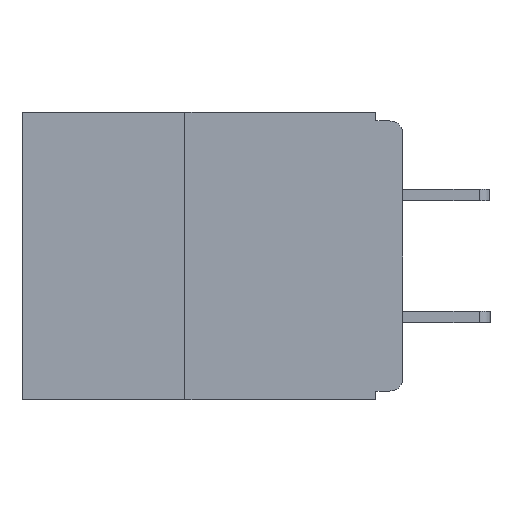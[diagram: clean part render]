
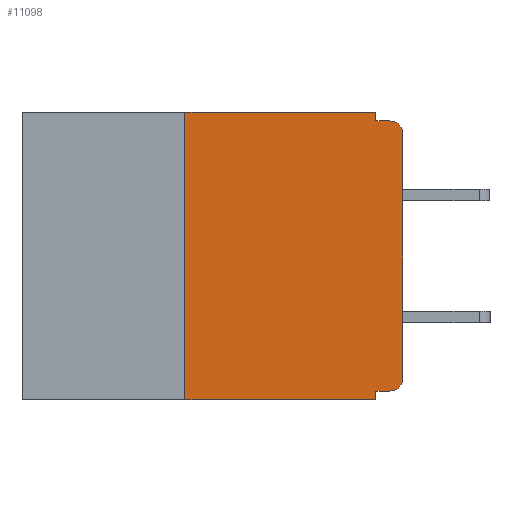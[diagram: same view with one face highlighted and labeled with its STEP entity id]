
A CAD part, left-side view. The second image highlights one B-rep face of the part: STEP entity #11098.
In plain terms, the highlighted planar face has unit normal (-1, 0, 0).
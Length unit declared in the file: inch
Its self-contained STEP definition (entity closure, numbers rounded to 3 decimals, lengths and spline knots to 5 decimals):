
#135 = VERTEX_POINT ( 'NONE', #15580 ) ;
#170 = CIRCLE ( 'NONE', #280, 0.015 ) ;
#195 = LINE ( 'NONE', #10995, #635 ) ;
#280 = AXIS2_PLACEMENT_3D ( 'NONE', #10115, #15134, #9453 ) ;
#335 = CARTESIAN_POINT ( 'NONE',  ( 0., 0., 0. ) ) ;
#342 = DIRECTION ( 'NONE',  ( 0., -1., 0. ) ) ;
#635 = VECTOR ( 'NONE', #12312, 39.37008 ) ;
#1055 = EDGE_CURVE ( 'NONE', #2756, #9159, #3602, .T. ) ;
#1391 = CARTESIAN_POINT ( 'NONE',  ( 0., 0.031, 0. ) ) ;
#1421 = DIRECTION ( 'NONE',  ( 0., 0., 1. ) ) ;
#2058 = CARTESIAN_POINT ( 'NONE',  ( 0., 0.25, 0. ) ) ;
#2737 = PLANE ( 'NONE',  #4023 ) ;
#2756 = VERTEX_POINT ( 'NONE', #2058 ) ;
#2779 = VECTOR ( 'NONE', #342, 39.37008 ) ;
#2857 = EDGE_CURVE ( 'NONE', #10114, #12999, #7992, .T. ) ;
#3011 = LINE ( 'NONE', #7369, #5942 ) ;
#3602 = LINE ( 'NONE', #5899, #2779 ) ;
#3689 = EDGE_CURVE ( 'NONE', #5447, #9240, #5818, .T. ) ;
#4023 = AXIS2_PLACEMENT_3D ( 'NONE', #8951, #11611, #4032 ) ;
#4032 = DIRECTION ( 'NONE',  ( 0., 0., -1. ) ) ;
#4285 = CARTESIAN_POINT ( 'NONE',  ( 0., 0.015, -0.01 ) ) ;
#4434 = EDGE_CURVE ( 'NONE', #10734, #10114, #4457, .T. ) ;
#4453 = DIRECTION ( 'NONE',  ( 0., 1., 0. ) ) ;
#4457 = CIRCLE ( 'NONE', #14322, 0.015 ) ;
#4703 = VECTOR ( 'NONE', #1421, 39.37008 ) ;
#4987 = ORIENTED_EDGE ( 'NONE', *, *, #5358, .T. ) ;
#5358 = EDGE_CURVE ( 'NONE', #12999, #9908, #170, .T. ) ;
#5366 = ORIENTED_EDGE ( 'NONE', *, *, #5831, .F. ) ;
#5447 = VERTEX_POINT ( 'NONE', #13940 ) ;
#5608 = EDGE_CURVE ( 'NONE', #135, #9908, #3011, .T. ) ;
#5724 = CARTESIAN_POINT ( 'NONE',  ( 0., 0.031, -0.32 ) ) ;
#5779 = ORIENTED_EDGE ( 'NONE', *, *, #3689, .T. ) ;
#5818 = LINE ( 'NONE', #7388, #12221 ) ;
#5831 = EDGE_CURVE ( 'NONE', #9159, #135, #6345, .T. ) ;
#5899 = CARTESIAN_POINT ( 'NONE',  ( 0., 0.437, 0. ) ) ;
#5942 = VECTOR ( 'NONE', #11221, 39.37008 ) ;
#6326 = LINE ( 'NONE', #8063, #6731 ) ;
#6345 = LINE ( 'NONE', #1391, #6525 ) ;
#6525 = VECTOR ( 'NONE', #8361, 39.37008 ) ;
#6533 = ORIENTED_EDGE ( 'NONE', *, *, #5608, .F. ) ;
#6731 = VECTOR ( 'NONE', #4453, 39.37008 ) ;
#7092 = CARTESIAN_POINT ( 'NONE',  ( 0., 0., -0.305 ) ) ;
#7369 = CARTESIAN_POINT ( 'NONE',  ( 0., 0., -0.01 ) ) ;
#7388 = CARTESIAN_POINT ( 'NONE',  ( 0., 0.437, -0.33 ) ) ;
#7427 = DIRECTION ( 'NONE',  ( 0., -1., 0. ) ) ;
#7992 = LINE ( 'NONE', #335, #4703 ) ;
#8063 = CARTESIAN_POINT ( 'NONE',  ( 0., 0., -0.32 ) ) ;
#8087 = ORIENTED_EDGE ( 'NONE', *, *, #2857, .T. ) ;
#8141 = ORIENTED_EDGE ( 'NONE', *, *, #14789, .F. ) ;
#8306 = EDGE_CURVE ( 'NONE', #10734, #14682, #6326, .T. ) ;
#8361 = DIRECTION ( 'NONE',  ( 0., 0., -1. ) ) ;
#8503 = ORIENTED_EDGE ( 'NONE', *, *, #1055, .F. ) ;
#8521 = ORIENTED_EDGE ( 'NONE', *, *, #8306, .F. ) ;
#8951 = CARTESIAN_POINT ( 'NONE',  ( 0., 0.437, 0. ) ) ;
#9159 = VERTEX_POINT ( 'NONE', #13870 ) ;
#9240 = VERTEX_POINT ( 'NONE', #11540 ) ;
#9453 = DIRECTION ( 'NONE',  ( 0., 0., -1. ) ) ;
#9908 = VERTEX_POINT ( 'NONE', #4285 ) ;
#10114 = VERTEX_POINT ( 'NONE', #7092 ) ;
#10115 = CARTESIAN_POINT ( 'NONE',  ( 0., 0.015, -0.025 ) ) ;
#10734 = VERTEX_POINT ( 'NONE', #15820 ) ;
#10995 = CARTESIAN_POINT ( 'NONE',  ( 0., 0.031, -0.33 ) ) ;
#11098 = ADVANCED_FACE ( 'NONE', ( #13429 ), #2737, .F. ) ;
#11179 = EDGE_CURVE ( 'NONE', #5447, #2756, #12275, .T. ) ;
#11221 = DIRECTION ( 'NONE',  ( 0., -1., 0. ) ) ;
#11540 = CARTESIAN_POINT ( 'NONE',  ( 0., 0.031, -0.33 ) ) ;
#11611 = DIRECTION ( 'NONE',  ( 1., 0., 0. ) ) ;
#12180 = ORIENTED_EDGE ( 'NONE', *, *, #11179, .F. ) ;
#12221 = VECTOR ( 'NONE', #7427, 39.37008 ) ;
#12275 = LINE ( 'NONE', #13033, #15164 ) ;
#12312 = DIRECTION ( 'NONE',  ( 0., 0., -1. ) ) ;
#12561 = CARTESIAN_POINT ( 'NONE',  ( 0., 0., -0.025 ) ) ;
#12999 = VERTEX_POINT ( 'NONE', #12561 ) ;
#13033 = CARTESIAN_POINT ( 'NONE',  ( 0., 0.25, -0.33 ) ) ;
#13429 = FACE_OUTER_BOUND ( 'NONE', #14368, .T. ) ;
#13870 = CARTESIAN_POINT ( 'NONE',  ( 0., 0.031, 0. ) ) ;
#13940 = CARTESIAN_POINT ( 'NONE',  ( 0., 0.25, -0.33 ) ) ;
#14279 = DIRECTION ( 'NONE',  ( 0., 0., 1. ) ) ;
#14322 = AXIS2_PLACEMENT_3D ( 'NONE', #16334, #16281, #16142 ) ;
#14338 = ORIENTED_EDGE ( 'NONE', *, *, #4434, .T. ) ;
#14368 = EDGE_LOOP ( 'NONE', ( #8087, #4987, #6533, #5366, #8503, #12180, #5779, #8141, #8521, #14338 ) ) ;
#14682 = VERTEX_POINT ( 'NONE', #5724 ) ;
#14789 = EDGE_CURVE ( 'NONE', #14682, #9240, #195, .T. ) ;
#15134 = DIRECTION ( 'NONE',  ( -1., 0., 0. ) ) ;
#15164 = VECTOR ( 'NONE', #14279, 39.37008 ) ;
#15580 = CARTESIAN_POINT ( 'NONE',  ( 0., 0.031, -0.01 ) ) ;
#15820 = CARTESIAN_POINT ( 'NONE',  ( 0., 0.015, -0.32 ) ) ;
#16142 = DIRECTION ( 'NONE',  ( 0., 0., -1. ) ) ;
#16281 = DIRECTION ( 'NONE',  ( -1., 0., 0. ) ) ;
#16334 = CARTESIAN_POINT ( 'NONE',  ( 0., 0.015, -0.305 ) ) ;
